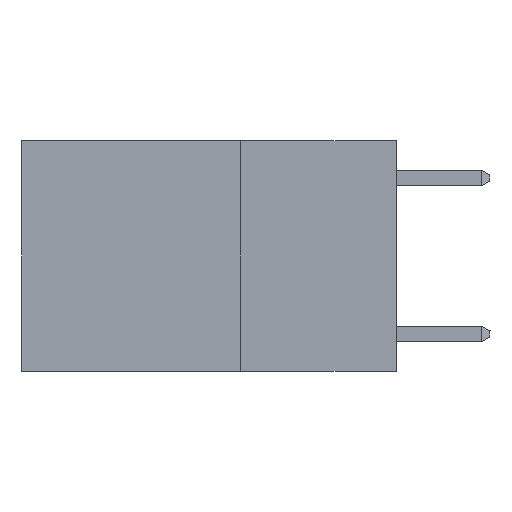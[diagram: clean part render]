
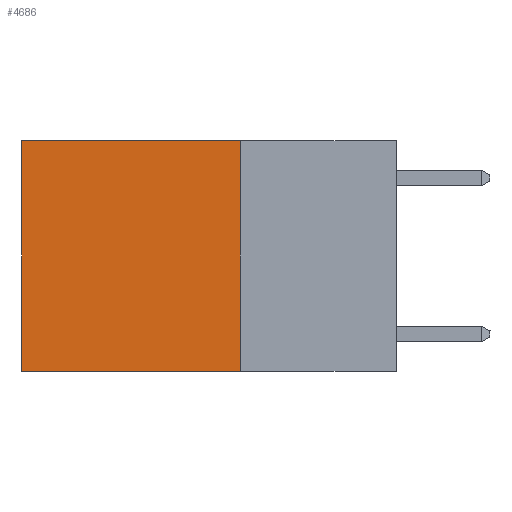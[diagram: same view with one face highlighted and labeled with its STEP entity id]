
A CAD part, left-side view. The second image highlights one B-rep face of the part: STEP entity #4686.
In plain terms, the highlighted planar face has unit normal (-1, 0, 0).
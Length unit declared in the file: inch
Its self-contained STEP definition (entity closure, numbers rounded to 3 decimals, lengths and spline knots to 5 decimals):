
#1377 = EDGE_CURVE ( 'NONE', #10460, #10532, #14263, .T. ) ;
#2297 = VECTOR ( 'NONE', #16440, 39.37008 ) ;
#2619 = DIRECTION ( 'NONE',  ( 0., 1., 0. ) ) ;
#2897 = CARTESIAN_POINT ( 'NONE',  ( 0.2625, 0.25, -0.37 ) ) ;
#3431 = VECTOR ( 'NONE', #9144, 39.37008 ) ;
#3992 = CARTESIAN_POINT ( 'NONE',  ( 0.2625, 0.25, 0. ) ) ;
#4024 = VERTEX_POINT ( 'NONE', #14040 ) ;
#4686 = ADVANCED_FACE ( 'NONE', ( #8414 ), #6918, .F. ) ;
#4728 = ORIENTED_EDGE ( 'NONE', *, *, #1377, .F. ) ;
#5217 = VECTOR ( 'NONE', #2619, 39.37008 ) ;
#6858 = EDGE_CURVE ( 'NONE', #10460, #11416, #8647, .T. ) ;
#6918 = PLANE ( 'NONE',  #13722 ) ;
#8223 = DIRECTION ( 'NONE',  ( 1., 0., 0. ) ) ;
#8414 = FACE_OUTER_BOUND ( 'NONE', #9231, .T. ) ;
#8628 = LINE ( 'NONE', #15432, #5217 ) ;
#8647 = LINE ( 'NONE', #3992, #3431 ) ;
#8966 = EDGE_CURVE ( 'NONE', #11416, #4024, #14348, .T. ) ;
#9144 = DIRECTION ( 'NONE',  ( 0., 1., 0. ) ) ;
#9231 = EDGE_LOOP ( 'NONE', ( #13249, #16105, #4728, #16279 ) ) ;
#10460 = VERTEX_POINT ( 'NONE', #11852 ) ;
#10532 = VERTEX_POINT ( 'NONE', #2897 ) ;
#11165 = CARTESIAN_POINT ( 'NONE',  ( 0.2625, 0.6, 0. ) ) ;
#11416 = VERTEX_POINT ( 'NONE', #11165 ) ;
#11852 = CARTESIAN_POINT ( 'NONE',  ( 0.2625, 0.25, 0. ) ) ;
#12068 = DIRECTION ( 'NONE',  ( 0., 0., -1. ) ) ;
#13141 = VECTOR ( 'NONE', #15523, 39.37008 ) ;
#13249 = ORIENTED_EDGE ( 'NONE', *, *, #8966, .T. ) ;
#13391 = EDGE_CURVE ( 'NONE', #10532, #4024, #8628, .T. ) ;
#13722 = AXIS2_PLACEMENT_3D ( 'NONE', #15872, #8223, #12068 ) ;
#13795 = CARTESIAN_POINT ( 'NONE',  ( 0.2625, 0.25, 0. ) ) ;
#14040 = CARTESIAN_POINT ( 'NONE',  ( 0.2625, 0.6, -0.37 ) ) ;
#14263 = LINE ( 'NONE', #13795, #2297 ) ;
#14266 = CARTESIAN_POINT ( 'NONE',  ( 0.2625, 0.6, 0. ) ) ;
#14348 = LINE ( 'NONE', #14266, #13141 ) ;
#15432 = CARTESIAN_POINT ( 'NONE',  ( 0.2625, 0.25, -0.37 ) ) ;
#15523 = DIRECTION ( 'NONE',  ( 0., 0., -1. ) ) ;
#15872 = CARTESIAN_POINT ( 'NONE',  ( 0.2625, 0.25, 0. ) ) ;
#16105 = ORIENTED_EDGE ( 'NONE', *, *, #13391, .F. ) ;
#16279 = ORIENTED_EDGE ( 'NONE', *, *, #6858, .T. ) ;
#16440 = DIRECTION ( 'NONE',  ( 0., 0., -1. ) ) ;
